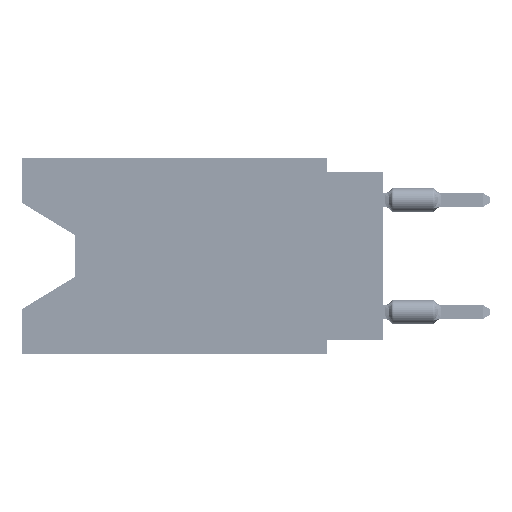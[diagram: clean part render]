
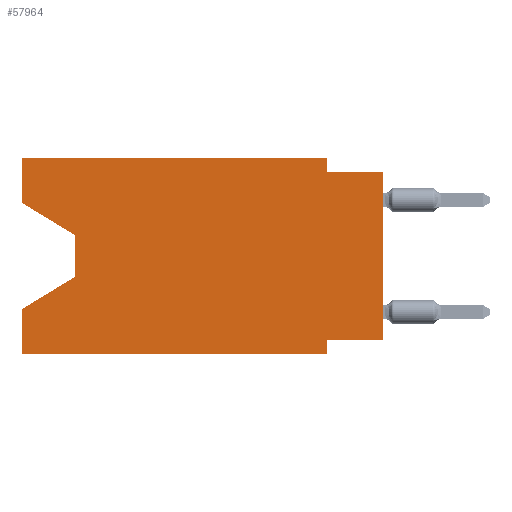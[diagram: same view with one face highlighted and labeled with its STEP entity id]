
A CAD part, left-side view. The second image highlights one B-rep face of the part: STEP entity #57964.
In plain terms, the highlighted planar face has unit normal (-1, 0, 0).
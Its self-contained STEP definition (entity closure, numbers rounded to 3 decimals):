
#1168 = EDGE_CURVE ( 'NONE', #42506, #57474, #1475, .T. ) ;
#1475 = LINE ( 'NONE', #20809, #48624 ) ;
#1940 = ORIENTED_EDGE ( 'NONE', *, *, #21423, .T. ) ;
#2101 = CARTESIAN_POINT ( 'NONE',  ( 0., 13.97, -3.505 ) ) ;
#2513 = LINE ( 'NONE', #71871, #50742 ) ;
#3891 = ORIENTED_EDGE ( 'NONE', *, *, #78471, .F. ) ;
#6663 = LINE ( 'NONE', #64236, #68428 ) ;
#7033 = VERTEX_POINT ( 'NONE', #46125 ) ;
#8077 = ORIENTED_EDGE ( 'NONE', *, *, #54482, .F. ) ;
#10221 = VECTOR ( 'NONE', #34893, 1000. ) ;
#11365 = DIRECTION ( 'NONE',  ( 0., -1., 0. ) ) ;
#11993 = CARTESIAN_POINT ( 'NONE',  ( 0., 2.54, -8.89 ) ) ;
#14137 = PLANE ( 'NONE',  #18764 ) ;
#14402 = CARTESIAN_POINT ( 'NONE',  ( 0., 16.383, -2.038 ) ) ;
#15106 = CARTESIAN_POINT ( 'NONE',  ( 0., 2.54, 0. ) ) ;
#15559 = VERTEX_POINT ( 'NONE', #25522 ) ;
#16106 = CARTESIAN_POINT ( 'NONE',  ( 0., 2.54, 0. ) ) ;
#16734 = CARTESIAN_POINT ( 'NONE',  ( 0., 13.97, -5.385 ) ) ;
#17319 = ORIENTED_EDGE ( 'NONE', *, *, #38288, .F. ) ;
#17530 = CARTESIAN_POINT ( 'NONE',  ( 0., 2.54, -8.89 ) ) ;
#17571 = VECTOR ( 'NONE', #28198, 1000. ) ;
#17794 = CARTESIAN_POINT ( 'NONE',  ( 0., 0., 0. ) ) ;
#18575 = CARTESIAN_POINT ( 'NONE',  ( 0., 16.383, -8.89 ) ) ;
#18764 = AXIS2_PLACEMENT_3D ( 'NONE', #22094, #80494, #79684 ) ;
#18865 = ORIENTED_EDGE ( 'NONE', *, *, #71367, .F. ) ;
#19641 = EDGE_CURVE ( 'NONE', #35519, #7033, #54977, .T. ) ;
#20442 = FACE_OUTER_BOUND ( 'NONE', #26708, .T. ) ;
#20809 = CARTESIAN_POINT ( 'NONE',  ( 0., 16.383, -2.038 ) ) ;
#21121 = VERTEX_POINT ( 'NONE', #36638 ) ;
#21221 = VECTOR ( 'NONE', #11365, 1000. ) ;
#21423 = EDGE_CURVE ( 'NONE', #57474, #35519, #73125, .T. ) ;
#22094 = CARTESIAN_POINT ( 'NONE',  ( 0., 16.383, 0. ) ) ;
#23248 = VERTEX_POINT ( 'NONE', #17530 ) ;
#23564 = LINE ( 'NONE', #67281, #17571 ) ;
#24211 = VERTEX_POINT ( 'NONE', #18575 ) ;
#25161 = DIRECTION ( 'NONE',  ( 0., 0., 1. ) ) ;
#25282 = EDGE_CURVE ( 'NONE', #38730, #65794, #23564, .T. ) ;
#25522 = CARTESIAN_POINT ( 'NONE',  ( 0., 2.54, -0.635 ) ) ;
#25963 = VECTOR ( 'NONE', #74723, 1000. ) ;
#26016 = CARTESIAN_POINT ( 'NONE',  ( 0., 13.97, -3.505 ) ) ;
#26708 = EDGE_LOOP ( 'NONE', ( #50369, #1940, #66738, #17319, #78406, #31475, #56624, #67513, #8077, #18865, #37021, #3891 ) ) ;
#27792 = EDGE_CURVE ( 'NONE', #21121, #74189, #43418, .T. ) ;
#28198 = DIRECTION ( 'NONE',  ( 0., 1., 0. ) ) ;
#28599 = VECTOR ( 'NONE', #44236, 1000. ) ;
#29586 = CARTESIAN_POINT ( 'NONE',  ( 0., 16.383, 0. ) ) ;
#31475 = ORIENTED_EDGE ( 'NONE', *, *, #62293, .F. ) ;
#34893 = DIRECTION ( 'NONE',  ( 0., 0., 1. ) ) ;
#35519 = VERTEX_POINT ( 'NONE', #65589 ) ;
#35770 = VECTOR ( 'NONE', #73738, 1000. ) ;
#36563 = VECTOR ( 'NONE', #60228, 1000. ) ;
#36638 = CARTESIAN_POINT ( 'NONE',  ( 0., 16.383, 0. ) ) ;
#36802 = DIRECTION ( 'NONE',  ( 0., 0., -1. ) ) ;
#37021 = ORIENTED_EDGE ( 'NONE', *, *, #27792, .F. ) ;
#37805 = LINE ( 'NONE', #74814, #21221 ) ;
#38288 = EDGE_CURVE ( 'NONE', #24211, #7033, #6663, .T. ) ;
#38730 = VERTEX_POINT ( 'NONE', #58540 ) ;
#40178 = VECTOR ( 'NONE', #53378, 1000. ) ;
#42506 = VERTEX_POINT ( 'NONE', #14402 ) ;
#43418 = LINE ( 'NONE', #61521, #28599 ) ;
#44236 = DIRECTION ( 'NONE',  ( 0., -1., 0. ) ) ;
#46125 = CARTESIAN_POINT ( 'NONE',  ( 0., 16.383, -6.852 ) ) ;
#46429 = DIRECTION ( 'NONE',  ( 0., -0.855, -0.519 ) ) ;
#48100 = LINE ( 'NONE', #29586, #35770 ) ;
#48624 = VECTOR ( 'NONE', #46429, 1000. ) ;
#49734 = LINE ( 'NONE', #17794, #10221 ) ;
#50369 = ORIENTED_EDGE ( 'NONE', *, *, #1168, .T. ) ;
#50742 = VECTOR ( 'NONE', #60078, 1000. ) ;
#53378 = DIRECTION ( 'NONE',  ( 0., 0., -1. ) ) ;
#53941 = LINE ( 'NONE', #16106, #36563 ) ;
#54482 = EDGE_CURVE ( 'NONE', #15559, #66216, #37805, .T. ) ;
#54977 = LINE ( 'NONE', #16734, #25963 ) ;
#56624 = ORIENTED_EDGE ( 'NONE', *, *, #25282, .F. ) ;
#57474 = VERTEX_POINT ( 'NONE', #26016 ) ;
#57964 = ADVANCED_FACE ( 'NONE', ( #20442 ), #14137, .F. ) ;
#58540 = CARTESIAN_POINT ( 'NONE',  ( 0., 0., -8.255 ) ) ;
#60078 = DIRECTION ( 'NONE',  ( 0., -1., 0. ) ) ;
#60228 = DIRECTION ( 'NONE',  ( 0., 0., -1. ) ) ;
#61521 = CARTESIAN_POINT ( 'NONE',  ( 0., 16.383, 0. ) ) ;
#62293 = EDGE_CURVE ( 'NONE', #65794, #23248, #82196, .T. ) ;
#64061 = EDGE_CURVE ( 'NONE', #38730, #66216, #49734, .T. ) ;
#64236 = CARTESIAN_POINT ( 'NONE',  ( 0., 16.383, 0. ) ) ;
#64946 = CARTESIAN_POINT ( 'NONE',  ( 0., 0., -0.635 ) ) ;
#65589 = CARTESIAN_POINT ( 'NONE',  ( 0., 13.97, -5.385 ) ) ;
#65794 = VERTEX_POINT ( 'NONE', #71351 ) ;
#66216 = VERTEX_POINT ( 'NONE', #64946 ) ;
#66371 = VECTOR ( 'NONE', #36802, 1000. ) ;
#66558 = EDGE_CURVE ( 'NONE', #24211, #23248, #2513, .T. ) ;
#66738 = ORIENTED_EDGE ( 'NONE', *, *, #19641, .T. ) ;
#67281 = CARTESIAN_POINT ( 'NONE',  ( 0., 0., -8.255 ) ) ;
#67513 = ORIENTED_EDGE ( 'NONE', *, *, #64061, .T. ) ;
#68428 = VECTOR ( 'NONE', #25161, 1000. ) ;
#71351 = CARTESIAN_POINT ( 'NONE',  ( 0., 2.54, -8.255 ) ) ;
#71367 = EDGE_CURVE ( 'NONE', #74189, #15559, #53941, .T. ) ;
#71871 = CARTESIAN_POINT ( 'NONE',  ( 0., 16.383, -8.89 ) ) ;
#73125 = LINE ( 'NONE', #2101, #40178 ) ;
#73738 = DIRECTION ( 'NONE',  ( 0., 0., 1. ) ) ;
#74189 = VERTEX_POINT ( 'NONE', #15106 ) ;
#74723 = DIRECTION ( 'NONE',  ( 0., 0.855, -0.519 ) ) ;
#74814 = CARTESIAN_POINT ( 'NONE',  ( 0., 0., -0.635 ) ) ;
#78406 = ORIENTED_EDGE ( 'NONE', *, *, #66558, .T. ) ;
#78471 = EDGE_CURVE ( 'NONE', #42506, #21121, #48100, .T. ) ;
#79684 = DIRECTION ( 'NONE',  ( 0., 0., -1. ) ) ;
#80494 = DIRECTION ( 'NONE',  ( 1., 0., 0. ) ) ;
#82196 = LINE ( 'NONE', #11993, #66371 ) ;
